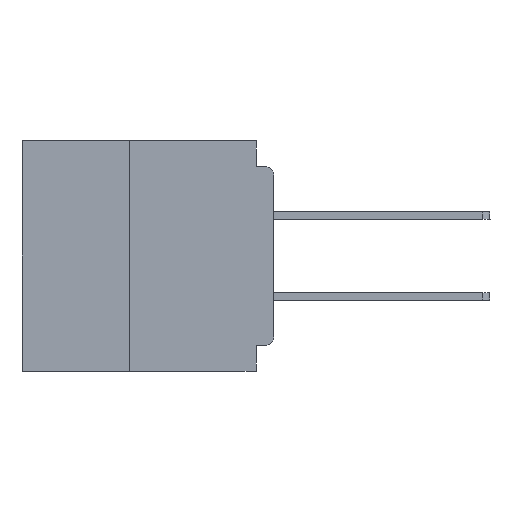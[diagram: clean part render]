
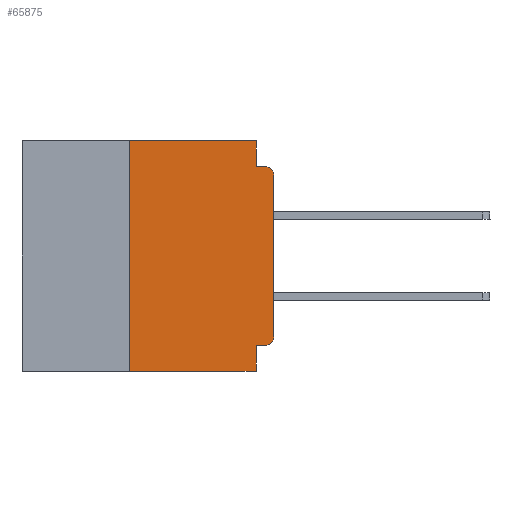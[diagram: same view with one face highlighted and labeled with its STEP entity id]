
A CAD part, left-side view. The second image highlights one B-rep face of the part: STEP entity #65875.
In plain terms, the highlighted planar face has unit normal (-1, 0, 0).
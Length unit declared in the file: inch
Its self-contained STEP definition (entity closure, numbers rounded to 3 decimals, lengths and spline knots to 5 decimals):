
#515 = DIRECTION ( 'NONE',  ( 0., -1., 0. ) ) ;
#920 = DIRECTION ( 'NONE',  ( -1., 0., 0. ) ) ;
#1050 = CARTESIAN_POINT ( 'NONE',  ( 0., 0.25, -0.4 ) ) ;
#1956 = AXIS2_PLACEMENT_3D ( 'NONE', #32441, #920, #37734 ) ;
#2582 = VECTOR ( 'NONE', #515, 39.37008 ) ;
#3062 = CARTESIAN_POINT ( 'NONE',  ( 0., 0.25, 0. ) ) ;
#4046 = DIRECTION ( 'NONE',  ( 0., -1., 0. ) ) ;
#6223 = ORIENTED_EDGE ( 'NONE', *, *, #33029, .F. ) ;
#7595 = CARTESIAN_POINT ( 'NONE',  ( 0., 0.015, -0.355 ) ) ;
#8971 = EDGE_CURVE ( 'NONE', #14892, #35664, #11965, .T. ) ;
#9459 = ORIENTED_EDGE ( 'NONE', *, *, #28724, .T. ) ;
#10331 = VECTOR ( 'NONE', #55870, 39.37008 ) ;
#11442 = VECTOR ( 'NONE', #60550, 39.37008 ) ;
#11765 = CARTESIAN_POINT ( 'NONE',  ( 0., 0.015, -0.34 ) ) ;
#11797 = EDGE_CURVE ( 'NONE', #42681, #48120, #20135, .T. ) ;
#11965 = LINE ( 'NONE', #40245, #10331 ) ;
#14892 = VERTEX_POINT ( 'NONE', #49401 ) ;
#15647 = EDGE_CURVE ( 'NONE', #49848, #53115, #41021, .T. ) ;
#15661 = VECTOR ( 'NONE', #4046, 39.37008 ) ;
#16291 = DIRECTION ( 'NONE',  ( 1., 0., 0. ) ) ;
#17076 = DIRECTION ( 'NONE',  ( 0., 0., -1. ) ) ;
#18281 = LINE ( 'NONE', #63486, #2582 ) ;
#18515 = CARTESIAN_POINT ( 'NONE',  ( 0., 0.031, 0. ) ) ;
#20135 = LINE ( 'NONE', #67879, #48095 ) ;
#20722 = VERTEX_POINT ( 'NONE', #7595 ) ;
#21129 = EDGE_LOOP ( 'NONE', ( #9459, #56961, #66896, #33182, #39947, #37491, #29049, #64376, #6223, #21628 ) ) ;
#21628 = ORIENTED_EDGE ( 'NONE', *, *, #50941, .T. ) ;
#22883 = DIRECTION ( 'NONE',  ( 0., 0., 1. ) ) ;
#25822 = VECTOR ( 'NONE', #22883, 39.37008 ) ;
#26697 = CARTESIAN_POINT ( 'NONE',  ( 0., 0., -0.355 ) ) ;
#27470 = LINE ( 'NONE', #38500, #25822 ) ;
#28724 = EDGE_CURVE ( 'NONE', #65403, #51486, #27470, .T. ) ;
#29049 = ORIENTED_EDGE ( 'NONE', *, *, #66529, .T. ) ;
#29617 = LINE ( 'NONE', #65306, #31262 ) ;
#31262 = VECTOR ( 'NONE', #33845, 39.37008 ) ;
#32441 = CARTESIAN_POINT ( 'NONE',  ( 0., 0.015, -0.06 ) ) ;
#33029 = EDGE_CURVE ( 'NONE', #20722, #14892, #33434, .T. ) ;
#33182 = ORIENTED_EDGE ( 'NONE', *, *, #15647, .F. ) ;
#33434 = LINE ( 'NONE', #26697, #61380 ) ;
#33535 = AXIS2_PLACEMENT_3D ( 'NONE', #47751, #16291, #53005 ) ;
#33845 = DIRECTION ( 'NONE',  ( 0., -1., 0. ) ) ;
#35577 = CARTESIAN_POINT ( 'NONE',  ( 0., 0., -0.045 ) ) ;
#35664 = VERTEX_POINT ( 'NONE', #51246 ) ;
#36447 = DIRECTION ( 'NONE',  ( 0., 0., 1. ) ) ;
#36825 = CARTESIAN_POINT ( 'NONE',  ( 0., 0., -0.06 ) ) ;
#37491 = ORIENTED_EDGE ( 'NONE', *, *, #11797, .F. ) ;
#37734 = DIRECTION ( 'NONE',  ( 0., 0., -1. ) ) ;
#38500 = CARTESIAN_POINT ( 'NONE',  ( 0., 0., 0. ) ) ;
#38556 = CARTESIAN_POINT ( 'NONE',  ( 0., 0.031, 0. ) ) ;
#39947 = ORIENTED_EDGE ( 'NONE', *, *, #51150, .F. ) ;
#40245 = CARTESIAN_POINT ( 'NONE',  ( 0., 0.031, -0.4 ) ) ;
#41021 = LINE ( 'NONE', #18515, #11442 ) ;
#42181 = FACE_OUTER_BOUND ( 'NONE', #21129, .T. ) ;
#42220 = PLANE ( 'NONE',  #33535 ) ;
#42681 = VERTEX_POINT ( 'NONE', #1050 ) ;
#43571 = LINE ( 'NONE', #35577, #15661 ) ;
#47751 = CARTESIAN_POINT ( 'NONE',  ( 0., 0.437, 0. ) ) ;
#48095 = VECTOR ( 'NONE', #36447, 39.37008 ) ;
#48120 = VERTEX_POINT ( 'NONE', #3062 ) ;
#48505 = AXIS2_PLACEMENT_3D ( 'NONE', #11765, #48528, #17076 ) ;
#48528 = DIRECTION ( 'NONE',  ( -1., 0., 0. ) ) ;
#49401 = CARTESIAN_POINT ( 'NONE',  ( 0., 0.031, -0.355 ) ) ;
#49848 = VERTEX_POINT ( 'NONE', #38556 ) ;
#50941 = EDGE_CURVE ( 'NONE', #20722, #65403, #56760, .T. ) ;
#51150 = EDGE_CURVE ( 'NONE', #48120, #49848, #29617, .T. ) ;
#51246 = CARTESIAN_POINT ( 'NONE',  ( 0., 0.031, -0.4 ) ) ;
#51486 = VERTEX_POINT ( 'NONE', #36825 ) ;
#53005 = DIRECTION ( 'NONE',  ( 0., 0., -1. ) ) ;
#53115 = VERTEX_POINT ( 'NONE', #62061 ) ;
#54541 = EDGE_CURVE ( 'NONE', #51486, #67185, #55952, .T. ) ;
#55870 = DIRECTION ( 'NONE',  ( 0., 0., -1. ) ) ;
#55952 = CIRCLE ( 'NONE', #1956, 0.015 ) ;
#56760 = CIRCLE ( 'NONE', #48505, 0.015 ) ;
#56961 = ORIENTED_EDGE ( 'NONE', *, *, #54541, .T. ) ;
#58173 = DIRECTION ( 'NONE',  ( 0., 1., 0. ) ) ;
#60550 = DIRECTION ( 'NONE',  ( 0., 0., -1. ) ) ;
#61097 = EDGE_CURVE ( 'NONE', #53115, #67185, #43571, .T. ) ;
#61380 = VECTOR ( 'NONE', #58173, 39.37008 ) ;
#62061 = CARTESIAN_POINT ( 'NONE',  ( 0., 0.031, -0.045 ) ) ;
#63486 = CARTESIAN_POINT ( 'NONE',  ( 0., 0.437, -0.4 ) ) ;
#64376 = ORIENTED_EDGE ( 'NONE', *, *, #8971, .F. ) ;
#64799 = CARTESIAN_POINT ( 'NONE',  ( 0., 0.015, -0.045 ) ) ;
#65306 = CARTESIAN_POINT ( 'NONE',  ( 0., 0.437, 0. ) ) ;
#65403 = VERTEX_POINT ( 'NONE', #67630 ) ;
#65875 = ADVANCED_FACE ( 'NONE', ( #42181 ), #42220, .F. ) ;
#66529 = EDGE_CURVE ( 'NONE', #42681, #35664, #18281, .T. ) ;
#66896 = ORIENTED_EDGE ( 'NONE', *, *, #61097, .F. ) ;
#67185 = VERTEX_POINT ( 'NONE', #64799 ) ;
#67630 = CARTESIAN_POINT ( 'NONE',  ( 0., 0., -0.34 ) ) ;
#67879 = CARTESIAN_POINT ( 'NONE',  ( 0., 0.25, -0.4 ) ) ;
